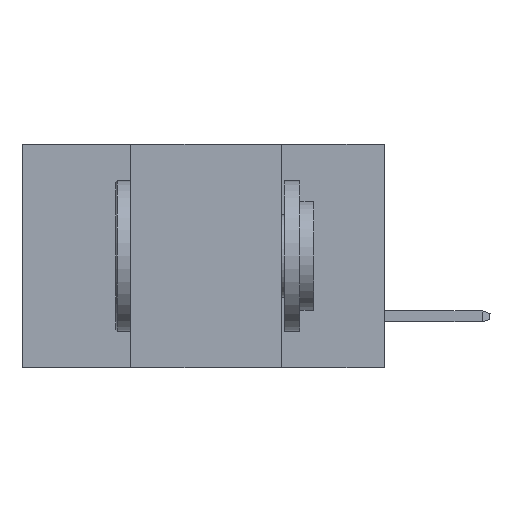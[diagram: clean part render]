
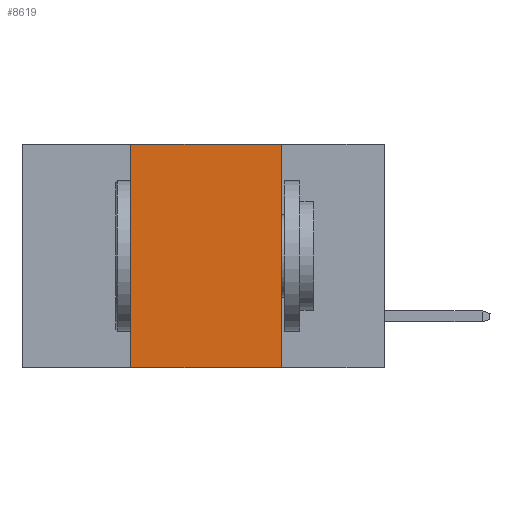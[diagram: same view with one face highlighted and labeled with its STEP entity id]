
A CAD part, left-side view. The second image highlights one B-rep face of the part: STEP entity #8619.
In plain terms, the highlighted planar face has unit normal (-1, 0, 0).
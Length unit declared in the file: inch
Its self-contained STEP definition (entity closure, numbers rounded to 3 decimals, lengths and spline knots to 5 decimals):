
#77 = VECTOR ( 'NONE', #8942, 39.37008 ) ;
#198 = DIRECTION ( 'NONE',  ( 0., 0., -1. ) ) ;
#1405 = ORIENTED_EDGE ( 'NONE', *, *, #4639, .F. ) ;
#2511 = EDGE_CURVE ( 'NONE', #8758, #14960, #10223, .T. ) ;
#2558 = CARTESIAN_POINT ( 'NONE',  ( 0., 0.42, 0. ) ) ;
#3189 = ORIENTED_EDGE ( 'NONE', *, *, #8781, .T. ) ;
#3521 = DIRECTION ( 'NONE',  ( 1., 0., 0. ) ) ;
#4639 = EDGE_CURVE ( 'NONE', #14960, #18173, #12240, .T. ) ;
#4795 = CARTESIAN_POINT ( 'NONE',  ( 0., 0.6, 0. ) ) ;
#5147 = VECTOR ( 'NONE', #13526, 39.37008 ) ;
#5206 = FACE_OUTER_BOUND ( 'NONE', #18103, .T. ) ;
#5882 = LINE ( 'NONE', #13325, #14163 ) ;
#6536 = VERTEX_POINT ( 'NONE', #9512 ) ;
#7462 = CARTESIAN_POINT ( 'NONE',  ( 0., 0.6, 0. ) ) ;
#8619 = ADVANCED_FACE ( 'NONE', ( #5206 ), #18494, .F. ) ;
#8758 = VERTEX_POINT ( 'NONE', #15870 ) ;
#8781 = EDGE_CURVE ( 'NONE', #8758, #6536, #5882, .T. ) ;
#8848 = CARTESIAN_POINT ( 'NONE',  ( 0., 0.42, -0.37 ) ) ;
#8942 = DIRECTION ( 'NONE',  ( 0., 0., 1. ) ) ;
#9109 = CARTESIAN_POINT ( 'NONE',  ( 0., 0.17, -0.37 ) ) ;
#9512 = CARTESIAN_POINT ( 'NONE',  ( 0., 0.17, -0.37 ) ) ;
#10223 = LINE ( 'NONE', #8848, #77 ) ;
#11209 = ORIENTED_EDGE ( 'NONE', *, *, #15217, .F. ) ;
#12240 = LINE ( 'NONE', #7462, #5147 ) ;
#13325 = CARTESIAN_POINT ( 'NONE',  ( 0., 0.6, -0.37 ) ) ;
#13526 = DIRECTION ( 'NONE',  ( 0., -1., 0. ) ) ;
#14163 = VECTOR ( 'NONE', #16242, 39.37008 ) ;
#14450 = ORIENTED_EDGE ( 'NONE', *, *, #2511, .F. ) ;
#14588 = VECTOR ( 'NONE', #198, 39.37008 ) ;
#14960 = VERTEX_POINT ( 'NONE', #2558 ) ;
#15217 = EDGE_CURVE ( 'NONE', #18173, #6536, #17815, .T. ) ;
#15870 = CARTESIAN_POINT ( 'NONE',  ( 0., 0.42, -0.37 ) ) ;
#16149 = CARTESIAN_POINT ( 'NONE',  ( 0., 0.17, 0. ) ) ;
#16242 = DIRECTION ( 'NONE',  ( 0., -1., 0. ) ) ;
#16645 = AXIS2_PLACEMENT_3D ( 'NONE', #4795, #3521, #17127 ) ;
#17127 = DIRECTION ( 'NONE',  ( 0., 0., -1. ) ) ;
#17815 = LINE ( 'NONE', #9109, #14588 ) ;
#18103 = EDGE_LOOP ( 'NONE', ( #11209, #1405, #14450, #3189 ) ) ;
#18173 = VERTEX_POINT ( 'NONE', #16149 ) ;
#18494 = PLANE ( 'NONE',  #16645 ) ;
